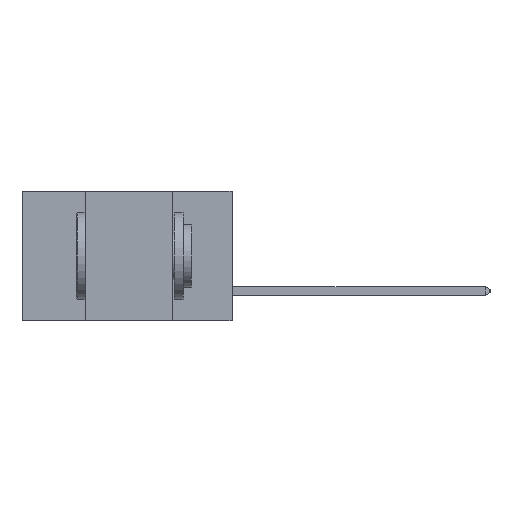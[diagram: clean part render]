
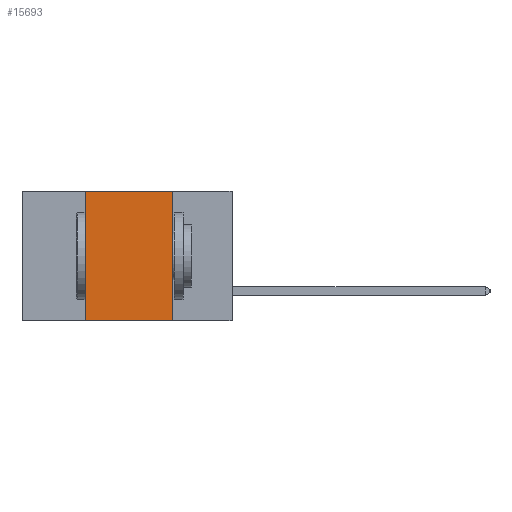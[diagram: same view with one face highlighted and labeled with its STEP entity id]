
A CAD part, left-side view. The second image highlights one B-rep face of the part: STEP entity #15693.
In plain terms, the highlighted planar face has unit normal (-1, 0, 0).
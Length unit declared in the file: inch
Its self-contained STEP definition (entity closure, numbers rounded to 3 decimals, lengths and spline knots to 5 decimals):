
#499 = VERTEX_POINT ( 'NONE', #6478 ) ;
#2529 = VERTEX_POINT ( 'NONE', #14366 ) ;
#2654 = EDGE_CURVE ( 'NONE', #499, #3477, #13048, .T. ) ;
#3145 = DIRECTION ( 'NONE',  ( 1., 0., 0. ) ) ;
#3223 = EDGE_CURVE ( 'NONE', #14853, #2529, #9006, .T. ) ;
#3239 = DIRECTION ( 'NONE',  ( 0., 0., -1. ) ) ;
#3477 = VERTEX_POINT ( 'NONE', #7730 ) ;
#3821 = CARTESIAN_POINT ( 'NONE',  ( 0., 0.17, 0. ) ) ;
#4488 = CARTESIAN_POINT ( 'NONE',  ( 0., 0.6, -0.37 ) ) ;
#5248 = VECTOR ( 'NONE', #3239, 39.37008 ) ;
#5250 = AXIS2_PLACEMENT_3D ( 'NONE', #14207, #3145, #11859 ) ;
#5348 = FACE_OUTER_BOUND ( 'NONE', #8013, .T. ) ;
#5725 = DIRECTION ( 'NONE',  ( 0., -1., 0. ) ) ;
#6156 = LINE ( 'NONE', #15388, #15569 ) ;
#6478 = CARTESIAN_POINT ( 'NONE',  ( 0., 0.42, -0.37 ) ) ;
#6823 = ORIENTED_EDGE ( 'NONE', *, *, #3223, .F. ) ;
#6977 = ORIENTED_EDGE ( 'NONE', *, *, #14514, .F. ) ;
#7102 = ORIENTED_EDGE ( 'NONE', *, *, #2654, .F. ) ;
#7166 = ORIENTED_EDGE ( 'NONE', *, *, #10390, .T. ) ;
#7730 = CARTESIAN_POINT ( 'NONE',  ( 0., 0.42, 0. ) ) ;
#8013 = EDGE_LOOP ( 'NONE', ( #6823, #6977, #7102, #7166 ) ) ;
#9006 = LINE ( 'NONE', #3821, #5248 ) ;
#9820 = VECTOR ( 'NONE', #13137, 39.37008 ) ;
#10390 = EDGE_CURVE ( 'NONE', #499, #2529, #11216, .T. ) ;
#10655 = PLANE ( 'NONE',  #5250 ) ;
#11216 = LINE ( 'NONE', #4488, #14010 ) ;
#11859 = DIRECTION ( 'NONE',  ( 0., 0., -1. ) ) ;
#12674 = CARTESIAN_POINT ( 'NONE',  ( 0., 0.17, 0. ) ) ;
#13048 = LINE ( 'NONE', #13218, #9820 ) ;
#13049 = DIRECTION ( 'NONE',  ( 0., -1., 0. ) ) ;
#13137 = DIRECTION ( 'NONE',  ( 0., 0., 1. ) ) ;
#13218 = CARTESIAN_POINT ( 'NONE',  ( 0., 0.42, 0. ) ) ;
#14010 = VECTOR ( 'NONE', #5725, 39.37008 ) ;
#14207 = CARTESIAN_POINT ( 'NONE',  ( 0., 0.6, 0. ) ) ;
#14366 = CARTESIAN_POINT ( 'NONE',  ( 0., 0.17, -0.37 ) ) ;
#14514 = EDGE_CURVE ( 'NONE', #3477, #14853, #6156, .T. ) ;
#14853 = VERTEX_POINT ( 'NONE', #12674 ) ;
#15388 = CARTESIAN_POINT ( 'NONE',  ( 0., 0.6, 0. ) ) ;
#15569 = VECTOR ( 'NONE', #13049, 39.37008 ) ;
#15693 = ADVANCED_FACE ( 'NONE', ( #5348 ), #10655, .F. ) ;
